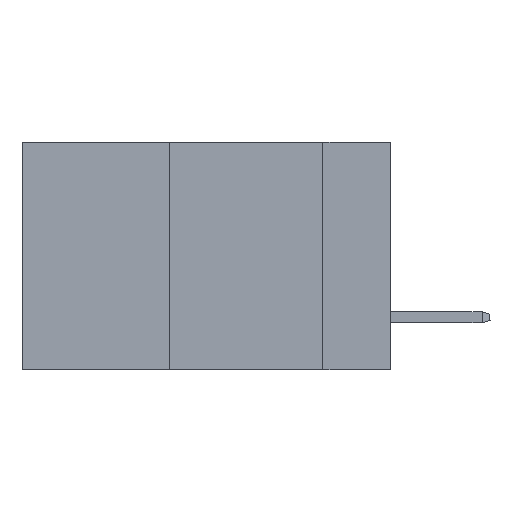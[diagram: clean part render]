
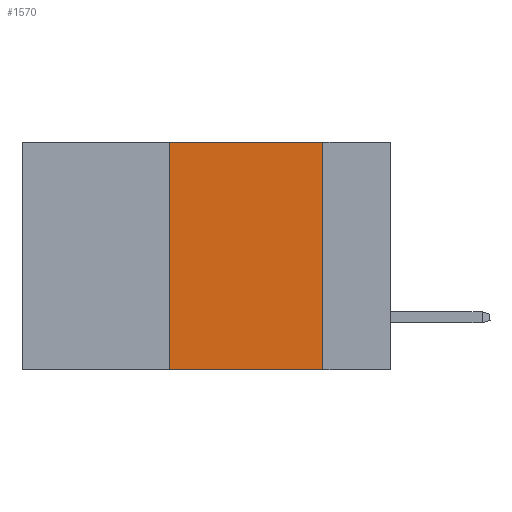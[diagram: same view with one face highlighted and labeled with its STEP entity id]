
A CAD part, left-side view. The second image highlights one B-rep face of the part: STEP entity #1570.
In plain terms, the highlighted planar face has unit normal (-1, 0, 0).
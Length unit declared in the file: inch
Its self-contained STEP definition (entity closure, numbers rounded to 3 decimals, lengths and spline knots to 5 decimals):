
#90 = CARTESIAN_POINT ( 'NONE',  ( 0., 0.6, -0.37 ) ) ;
#418 = CARTESIAN_POINT ( 'NONE',  ( 0., 0.11, 0. ) ) ;
#434 = EDGE_LOOP ( 'NONE', ( #6831, #3031, #6545, #8279 ) ) ;
#912 = DIRECTION ( 'NONE',  ( 0., -1., 0. ) ) ;
#968 = VECTOR ( 'NONE', #4538, 39.37008 ) ;
#1570 = ADVANCED_FACE ( 'NONE', ( #10035 ), #4621, .F. ) ;
#1990 = CARTESIAN_POINT ( 'NONE',  ( 0., 0.36, 0. ) ) ;
#2110 = EDGE_CURVE ( 'NONE', #7519, #4804, #3315, .T. ) ;
#2789 = CARTESIAN_POINT ( 'NONE',  ( 0., 0.36, -0.37 ) ) ;
#2867 = DIRECTION ( 'NONE',  ( 1., 0., 0. ) ) ;
#3031 = ORIENTED_EDGE ( 'NONE', *, *, #7489, .F. ) ;
#3315 = LINE ( 'NONE', #8086, #968 ) ;
#3788 = CARTESIAN_POINT ( 'NONE',  ( 0., 0.6, 0. ) ) ;
#3821 = EDGE_CURVE ( 'NONE', #6145, #7114, #9019, .T. ) ;
#4292 = CARTESIAN_POINT ( 'NONE',  ( 0., 0.36, 0. ) ) ;
#4538 = DIRECTION ( 'NONE',  ( 0., 0., -1. ) ) ;
#4621 = PLANE ( 'NONE',  #6432 ) ;
#4760 = VECTOR ( 'NONE', #6714, 39.37008 ) ;
#4804 = VERTEX_POINT ( 'NONE', #8180 ) ;
#5770 = EDGE_CURVE ( 'NONE', #6145, #4804, #6064, .T. ) ;
#6064 = LINE ( 'NONE', #90, #9216 ) ;
#6145 = VERTEX_POINT ( 'NONE', #2789 ) ;
#6432 = AXIS2_PLACEMENT_3D ( 'NONE', #3788, #2867, #8213 ) ;
#6545 = ORIENTED_EDGE ( 'NONE', *, *, #3821, .F. ) ;
#6714 = DIRECTION ( 'NONE',  ( 0., -1., 0. ) ) ;
#6831 = ORIENTED_EDGE ( 'NONE', *, *, #2110, .F. ) ;
#7099 = LINE ( 'NONE', #8421, #4760 ) ;
#7114 = VERTEX_POINT ( 'NONE', #4292 ) ;
#7367 = VECTOR ( 'NONE', #9739, 39.37008 ) ;
#7489 = EDGE_CURVE ( 'NONE', #7114, #7519, #7099, .T. ) ;
#7519 = VERTEX_POINT ( 'NONE', #418 ) ;
#8086 = CARTESIAN_POINT ( 'NONE',  ( 0., 0.11, 0. ) ) ;
#8180 = CARTESIAN_POINT ( 'NONE',  ( 0., 0.11, -0.37 ) ) ;
#8213 = DIRECTION ( 'NONE',  ( 0., 0., -1. ) ) ;
#8279 = ORIENTED_EDGE ( 'NONE', *, *, #5770, .T. ) ;
#8421 = CARTESIAN_POINT ( 'NONE',  ( 0., 0.6, 0. ) ) ;
#9019 = LINE ( 'NONE', #1990, #7367 ) ;
#9216 = VECTOR ( 'NONE', #912, 39.37008 ) ;
#9739 = DIRECTION ( 'NONE',  ( 0., 0., 1. ) ) ;
#10035 = FACE_OUTER_BOUND ( 'NONE', #434, .T. ) ;
